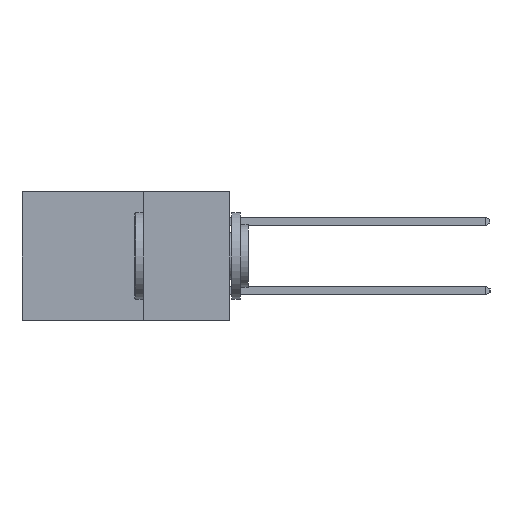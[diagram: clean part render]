
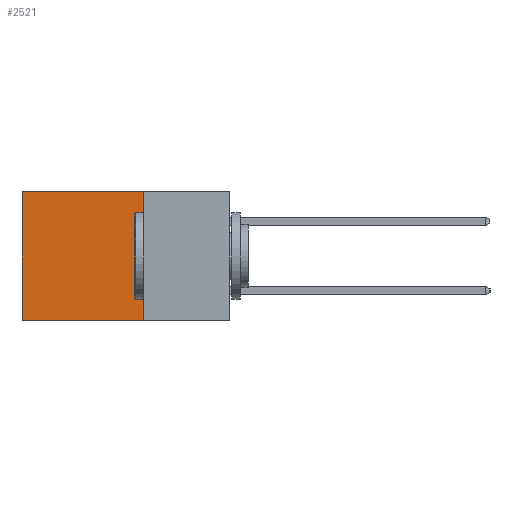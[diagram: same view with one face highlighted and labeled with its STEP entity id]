
A CAD part, left-side view. The second image highlights one B-rep face of the part: STEP entity #2521.
In plain terms, the highlighted planar face has unit normal (-1, 0, 0).
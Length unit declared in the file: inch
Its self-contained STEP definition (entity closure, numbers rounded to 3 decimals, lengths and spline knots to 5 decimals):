
#888 = CARTESIAN_POINT ( 'NONE',  ( 0.2615, 0.25, -0.37 ) ) ;
#2521 = ADVANCED_FACE ( 'NONE', ( #3346 ), #7106, .F. ) ;
#2666 = DIRECTION ( 'NONE',  ( 0., 1., 0. ) ) ;
#2714 = VERTEX_POINT ( 'NONE', #19185 ) ;
#3346 = FACE_OUTER_BOUND ( 'NONE', #9623, .T. ) ;
#4292 = EDGE_CURVE ( 'NONE', #16948, #6804, #17790, .T. ) ;
#4352 = DIRECTION ( 'NONE',  ( 0., 0., -1. ) ) ;
#5184 = DIRECTION ( 'NONE',  ( 0., 1., 0. ) ) ;
#5278 = EDGE_CURVE ( 'NONE', #16948, #2714, #19562, .T. ) ;
#5426 = VECTOR ( 'NONE', #2666, 39.37008 ) ;
#5970 = LINE ( 'NONE', #21141, #5426 ) ;
#6470 = VERTEX_POINT ( 'NONE', #8639 ) ;
#6804 = VERTEX_POINT ( 'NONE', #9412 ) ;
#7106 = PLANE ( 'NONE',  #13403 ) ;
#7749 = ORIENTED_EDGE ( 'NONE', *, *, #18846, .F. ) ;
#8639 = CARTESIAN_POINT ( 'NONE',  ( 0.2615, 0.6, -0.37 ) ) ;
#8799 = DIRECTION ( 'NONE',  ( 0., 0., -1. ) ) ;
#9412 = CARTESIAN_POINT ( 'NONE',  ( 0.2615, 0.25, -0.37 ) ) ;
#9623 = EDGE_LOOP ( 'NONE', ( #10902, #7749, #13733, #18510 ) ) ;
#10902 = ORIENTED_EDGE ( 'NONE', *, *, #19442, .T. ) ;
#12867 = VECTOR ( 'NONE', #14653, 39.37008 ) ;
#13403 = AXIS2_PLACEMENT_3D ( 'NONE', #17116, #18762, #8799 ) ;
#13733 = ORIENTED_EDGE ( 'NONE', *, *, #4292, .F. ) ;
#14653 = DIRECTION ( 'NONE',  ( 0., 0., -1. ) ) ;
#15168 = VECTOR ( 'NONE', #5184, 39.37008 ) ;
#16168 = CARTESIAN_POINT ( 'NONE',  ( 0.2615, 0.6, -0.37 ) ) ;
#16948 = VERTEX_POINT ( 'NONE', #18019 ) ;
#17116 = CARTESIAN_POINT ( 'NONE',  ( 0.2615, 0.25, -0.37 ) ) ;
#17225 = LINE ( 'NONE', #16168, #21600 ) ;
#17790 = LINE ( 'NONE', #888, #12867 ) ;
#18019 = CARTESIAN_POINT ( 'NONE',  ( 0.2615, 0.25, 0. ) ) ;
#18510 = ORIENTED_EDGE ( 'NONE', *, *, #5278, .T. ) ;
#18762 = DIRECTION ( 'NONE',  ( 1., 0., 0. ) ) ;
#18846 = EDGE_CURVE ( 'NONE', #6804, #6470, #5970, .T. ) ;
#19185 = CARTESIAN_POINT ( 'NONE',  ( 0.2615, 0.6, 0. ) ) ;
#19442 = EDGE_CURVE ( 'NONE', #2714, #6470, #17225, .T. ) ;
#19562 = LINE ( 'NONE', #21834, #15168 ) ;
#21141 = CARTESIAN_POINT ( 'NONE',  ( 0.2615, 0.25, -0.37 ) ) ;
#21600 = VECTOR ( 'NONE', #4352, 39.37008 ) ;
#21834 = CARTESIAN_POINT ( 'NONE',  ( 0.2615, 0.25, 0. ) ) ;
